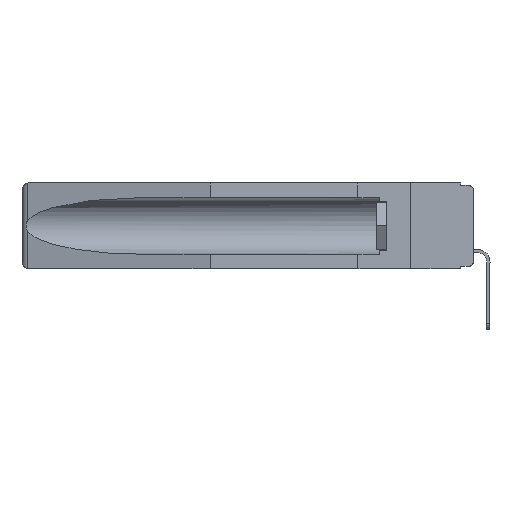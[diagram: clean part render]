
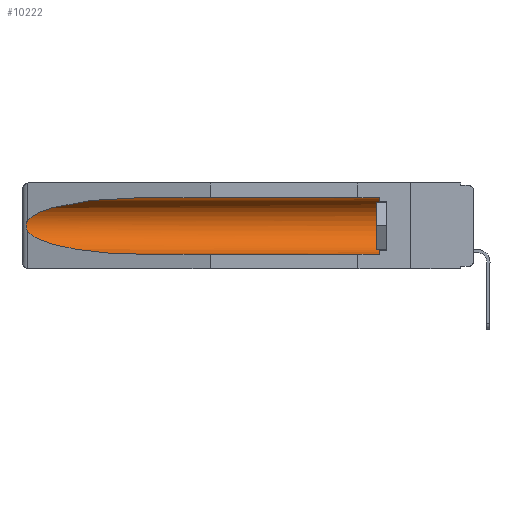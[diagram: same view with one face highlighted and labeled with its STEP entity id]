
A CAD part, left-side view. The second image highlights one B-rep face of the part: STEP entity #10222.
In plain terms, the highlighted cylindrical face has radius 2.857 mm (diameter 5.715 mm), a partial arc.
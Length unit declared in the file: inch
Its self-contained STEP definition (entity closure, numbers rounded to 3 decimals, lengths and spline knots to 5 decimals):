
#273 = EDGE_LOOP ( 'NONE', ( #4779, #7207, #5041, #9805, #15446, #15926 ) ) ;
#1365 = VECTOR ( 'NONE', #7938, 39.37008 ) ;
#1930 = CARTESIAN_POINT ( 'NONE',  ( 0.26597, 1.52961, -0.15275 ) ) ;
#1978 = CARTESIAN_POINT ( 'NONE',  ( 0.155, 0.126, -0.1715 ) ) ;
#2145 = CARTESIAN_POINT ( 'NONE',  ( 0.26537, 1.52718, -0.19328 ) ) ;
#2614 = VERTEX_POINT ( 'NONE', #12666 ) ;
#2787 = CARTESIAN_POINT ( 'NONE',  ( 0.155, 1.07973, -0.284 ) ) ;
#3772 = VERTEX_POINT ( 'NONE', #13726 ) ;
#3820 = CARTESIAN_POINT ( 'NONE',  ( 0.2673, 1.5327, -0.16383 ) ) ;
#4441 = CARTESIAN_POINT ( 'NONE',  ( 0.155, -0.30754, -0.284 ) ) ;
#4608 = CARTESIAN_POINT ( 'NONE',  ( 0.26537, 1.52718, -0.14972 ) ) ;
#4779 = ORIENTED_EDGE ( 'NONE', *, *, #17298, .T. ) ;
#5041 = ORIENTED_EDGE ( 'NONE', *, *, #12029, .T. ) ;
#5203 = CARTESIAN_POINT ( 'NONE',  ( 0.2675, 1.53308, -0.17534 ) ) ;
#5309 = CARTESIAN_POINT ( 'NONE',  ( 0.26655, 1.53094, -0.18657 ) ) ;
#5556 = LINE ( 'NONE', #13553, #15192 ) ;
#5909 =( BOUNDED_CURVE ( )  B_SPLINE_CURVE ( 3, ( #14065, #9374, #17452, #2787 ),
 .UNSPECIFIED., .F., .F. ) 
 B_SPLINE_CURVE_WITH_KNOTS ( ( 4, 4 ),
 ( 0.1948, 1.5708 ),
 .UNSPECIFIED. ) 
 CURVE ( )  GEOMETRIC_REPRESENTATION_ITEM ( )  RATIONAL_B_SPLINE_CURVE ( ( 1., 0.848, 0.848, 1. ) ) 
 REPRESENTATION_ITEM ( '' )  );
#5960 = AXIS2_PLACEMENT_3D ( 'NONE', #7160, #12186, #16730 ) ;
#6356 = VERTEX_POINT ( 'NONE', #17538 ) ;
#6955 = FACE_OUTER_BOUND ( 'NONE', #273, .T. ) ;
#7160 = CARTESIAN_POINT ( 'NONE',  ( 0.155, -0.30754, -0.1715 ) ) ;
#7207 = ORIENTED_EDGE ( 'NONE', *, *, #9833, .T. ) ;
#7938 = DIRECTION ( 'NONE',  ( 0., 1., 0. ) ) ;
#8493 = CARTESIAN_POINT ( 'NONE',  ( 0.26537, 1.52718, -0.14972 ) ) ;
#9374 = CARTESIAN_POINT ( 'NONE',  ( 0.25451, 1.48313, -0.24835 ) ) ;
#9727 = DIRECTION ( 'NONE',  ( 0., 0., 1. ) ) ;
#9805 = ORIENTED_EDGE ( 'NONE', *, *, #13382, .F. ) ;
#9833 = EDGE_CURVE ( 'NONE', #3772, #6356, #15537, .T. ) ;
#10144 = DIRECTION ( 'NONE',  ( 0., -1., 0. ) ) ;
#10222 = ADVANCED_FACE ( 'NONE', ( #6955 ), #10269, .F. ) ;
#10269 = CYLINDRICAL_SURFACE ( 'NONE', #5960, 0.1125 ) ;
#11330 = CARTESIAN_POINT ( 'NONE',  ( 0.155, 1.07973, -0.059 ) ) ;
#12029 = EDGE_CURVE ( 'NONE', #6356, #16002, #5909, .T. ) ;
#12186 = DIRECTION ( 'NONE',  ( 0., 1., 0. ) ) ;
#12666 = CARTESIAN_POINT ( 'NONE',  ( 0.155, 0.126, -0.059 ) ) ;
#12711 = CARTESIAN_POINT ( 'NONE',  ( 0.21114, 1.30732, -0.059 ) ) ;
#13199 = EDGE_CURVE ( 'NONE', #2614, #17340, #5556, .T. ) ;
#13264 = CIRCLE ( 'NONE', #20695, 0.1125 ) ;
#13382 = EDGE_CURVE ( 'NONE', #15988, #16002, #15704, .T. ) ;
#13553 = CARTESIAN_POINT ( 'NONE',  ( 0.155, -0.30754, -0.059 ) ) ;
#13726 = CARTESIAN_POINT ( 'NONE',  ( 0.26537, 1.52718, -0.14972 ) ) ;
#14065 = CARTESIAN_POINT ( 'NONE',  ( 0.26537, 1.52718, -0.19328 ) ) ;
#14985 = CARTESIAN_POINT ( 'NONE',  ( 0.2675, 1.53308, -0.16763 ) ) ;
#15192 = VECTOR ( 'NONE', #18117, 39.37008 ) ;
#15228 = EDGE_CURVE ( 'NONE', #15988, #2614, #13264, .T. ) ;
#15446 = ORIENTED_EDGE ( 'NONE', *, *, #15228, .T. ) ;
#15537 = B_SPLINE_CURVE_WITH_KNOTS ( 'NONE', 3,
 ( #8493, #1930, #19749, #3820, #14985, #5203, #19855, #5309, #16678, #2145 ),
 .UNSPECIFIED., .F., .F.,
 ( 4, 2, 2, 2, 4 ),
 ( 0., 0.00029, 0.00058, 0.00087, 0.00117 ),
 .UNSPECIFIED. ) ;
#15704 = LINE ( 'NONE', #4441, #1365 ) ;
#15926 = ORIENTED_EDGE ( 'NONE', *, *, #13199, .T. ) ;
#15988 = VERTEX_POINT ( 'NONE', #16032 ) ;
#16002 = VERTEX_POINT ( 'NONE', #19105 ) ;
#16032 = CARTESIAN_POINT ( 'NONE',  ( 0.155, 0.126, -0.284 ) ) ;
#16678 = CARTESIAN_POINT ( 'NONE',  ( 0.26597, 1.5296, -0.19026 ) ) ;
#16730 = DIRECTION ( 'NONE',  ( 0., 0., 1. ) ) ;
#16771 =( BOUNDED_CURVE ( )  B_SPLINE_CURVE ( 3, ( #11330, #12711, #19368, #4608 ),
 .UNSPECIFIED., .F., .F. ) 
 B_SPLINE_CURVE_WITH_KNOTS ( ( 4, 4 ),
 ( 4.71239, 6.08839 ),
 .UNSPECIFIED. ) 
 CURVE ( )  GEOMETRIC_REPRESENTATION_ITEM ( )  RATIONAL_B_SPLINE_CURVE ( ( 1., 0.848, 0.848, 1. ) ) 
 REPRESENTATION_ITEM ( '' )  );
#17298 = EDGE_CURVE ( 'NONE', #17340, #3772, #16771, .T. ) ;
#17340 = VERTEX_POINT ( 'NONE', #19268 ) ;
#17452 = CARTESIAN_POINT ( 'NONE',  ( 0.21114, 1.30732, -0.284 ) ) ;
#17538 = CARTESIAN_POINT ( 'NONE',  ( 0.26537, 1.52718, -0.19328 ) ) ;
#18117 = DIRECTION ( 'NONE',  ( 0., 1., 0. ) ) ;
#19105 = CARTESIAN_POINT ( 'NONE',  ( 0.155, 1.07973, -0.284 ) ) ;
#19268 = CARTESIAN_POINT ( 'NONE',  ( 0.155, 1.07973, -0.059 ) ) ;
#19368 = CARTESIAN_POINT ( 'NONE',  ( 0.25451, 1.48313, -0.09465 ) ) ;
#19749 = CARTESIAN_POINT ( 'NONE',  ( 0.26654, 1.53092, -0.15636 ) ) ;
#19855 = CARTESIAN_POINT ( 'NONE',  ( 0.2673, 1.53269, -0.17917 ) ) ;
#20695 = AXIS2_PLACEMENT_3D ( 'NONE', #1978, #10144, #9727 ) ;
